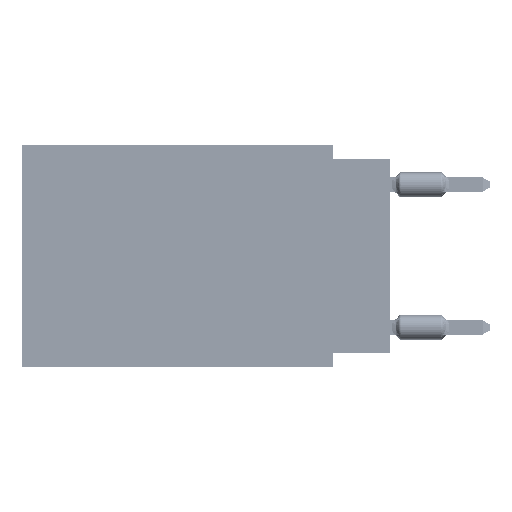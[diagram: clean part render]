
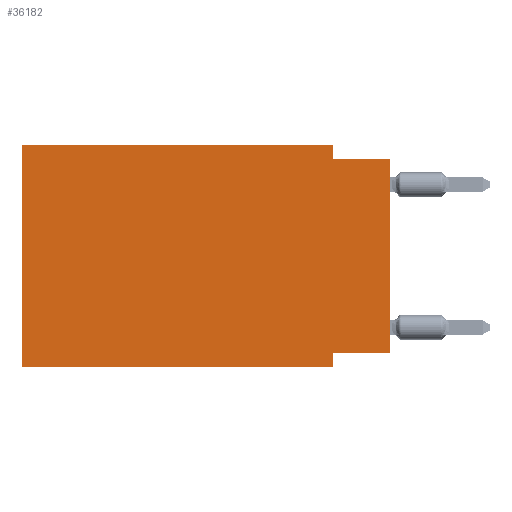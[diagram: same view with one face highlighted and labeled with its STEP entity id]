
A CAD part, left-side view. The second image highlights one B-rep face of the part: STEP entity #36182.
In plain terms, the highlighted planar face has unit normal (-1, 0, 0).
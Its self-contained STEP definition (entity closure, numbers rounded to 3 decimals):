
#5385 = CARTESIAN_POINT ( 'NONE',  ( 0., 2.54, 0. ) ) ;
#5853 = CARTESIAN_POINT ( 'NONE',  ( 0., 2.54, -9.906 ) ) ;
#7434 = EDGE_CURVE ( 'NONE', #43690, #29372, #51455, .T. ) ;
#8246 = DIRECTION ( 'NONE',  ( 0., 0., 1. ) ) ;
#9628 = DIRECTION ( 'NONE',  ( 0., 0., -1. ) ) ;
#9829 = EDGE_CURVE ( 'NONE', #29372, #57507, #38888, .T. ) ;
#11429 = EDGE_CURVE ( 'NONE', #43690, #33836, #52898, .T. ) ;
#11739 = CARTESIAN_POINT ( 'NONE',  ( 0., 16.383, 0. ) ) ;
#12144 = VERTEX_POINT ( 'NONE', #11739 ) ;
#13014 = VECTOR ( 'NONE', #66221, 1000. ) ;
#13335 = CARTESIAN_POINT ( 'NONE',  ( 0., 0., 0. ) ) ;
#14110 = DIRECTION ( 'NONE',  ( 0., -1., 0. ) ) ;
#15121 = VECTOR ( 'NONE', #14110, 1000. ) ;
#18585 = CARTESIAN_POINT ( 'NONE',  ( 0., 0., -9.271 ) ) ;
#19165 = VECTOR ( 'NONE', #28379, 1000. ) ;
#19522 = EDGE_CURVE ( 'NONE', #37060, #12144, #24349, .T. ) ;
#20546 = PLANE ( 'NONE',  #21403 ) ;
#20905 = ORIENTED_EDGE ( 'NONE', *, *, #7434, .F. ) ;
#21243 = VECTOR ( 'NONE', #57749, 1000. ) ;
#21403 = AXIS2_PLACEMENT_3D ( 'NONE', #70677, #31434, #9628 ) ;
#22285 = ORIENTED_EDGE ( 'NONE', *, *, #19522, .F. ) ;
#23385 = CARTESIAN_POINT ( 'NONE',  ( 0., 2.54, -0.635 ) ) ;
#24349 = LINE ( 'NONE', #35574, #21243 ) ;
#24928 = CARTESIAN_POINT ( 'NONE',  ( 0., 0., -0.635 ) ) ;
#26258 = VECTOR ( 'NONE', #8246, 1000. ) ;
#28379 = DIRECTION ( 'NONE',  ( 0., 0., -1. ) ) ;
#29372 = VERTEX_POINT ( 'NONE', #41130 ) ;
#31434 = DIRECTION ( 'NONE',  ( 1., 0., 0. ) ) ;
#33836 = VERTEX_POINT ( 'NONE', #62735 ) ;
#35095 = LINE ( 'NONE', #24928, #41537 ) ;
#35574 = CARTESIAN_POINT ( 'NONE',  ( 0., 16.383, 0. ) ) ;
#36182 = ADVANCED_FACE ( 'NONE', ( #53917 ), #20546, .F. ) ;
#37060 = VERTEX_POINT ( 'NONE', #42763 ) ;
#37344 = EDGE_CURVE ( 'NONE', #52095, #33836, #35095, .T. ) ;
#37492 = CARTESIAN_POINT ( 'NONE',  ( 0., 16.383, -9.906 ) ) ;
#37739 = ORIENTED_EDGE ( 'NONE', *, *, #9829, .F. ) ;
#38888 = LINE ( 'NONE', #5853, #19165 ) ;
#38912 = ORIENTED_EDGE ( 'NONE', *, *, #11429, .T. ) ;
#39270 = VERTEX_POINT ( 'NONE', #5385 ) ;
#41130 = CARTESIAN_POINT ( 'NONE',  ( 0., 2.54, -9.271 ) ) ;
#41537 = VECTOR ( 'NONE', #57251, 1000. ) ;
#41692 = LINE ( 'NONE', #63887, #15121 ) ;
#42763 = CARTESIAN_POINT ( 'NONE',  ( 0., 16.383, -9.906 ) ) ;
#43278 = DIRECTION ( 'NONE',  ( 0., -1., 0. ) ) ;
#43416 = EDGE_CURVE ( 'NONE', #37060, #57507, #59308, .T. ) ;
#43690 = VERTEX_POINT ( 'NONE', #18585 ) ;
#44213 = VECTOR ( 'NONE', #43278, 1000. ) ;
#46119 = ORIENTED_EDGE ( 'NONE', *, *, #54803, .F. ) ;
#47237 = CARTESIAN_POINT ( 'NONE',  ( 0., 2.54, -9.906 ) ) ;
#47550 = ORIENTED_EDGE ( 'NONE', *, *, #57164, .F. ) ;
#51119 = CARTESIAN_POINT ( 'NONE',  ( 0., 0., -9.271 ) ) ;
#51455 = LINE ( 'NONE', #51119, #61287 ) ;
#51520 = ORIENTED_EDGE ( 'NONE', *, *, #37344, .F. ) ;
#52095 = VERTEX_POINT ( 'NONE', #23385 ) ;
#52898 = LINE ( 'NONE', #13335, #26258 ) ;
#53917 = FACE_OUTER_BOUND ( 'NONE', #66120, .T. ) ;
#54803 = EDGE_CURVE ( 'NONE', #12144, #39270, #41692, .T. ) ;
#57164 = EDGE_CURVE ( 'NONE', #39270, #52095, #61468, .T. ) ;
#57251 = DIRECTION ( 'NONE',  ( 0., -1., 0. ) ) ;
#57507 = VERTEX_POINT ( 'NONE', #47237 ) ;
#57749 = DIRECTION ( 'NONE',  ( 0., 0., 1. ) ) ;
#59308 = LINE ( 'NONE', #37492, #44213 ) ;
#61285 = ORIENTED_EDGE ( 'NONE', *, *, #43416, .T. ) ;
#61287 = VECTOR ( 'NONE', #68920, 1000. ) ;
#61468 = LINE ( 'NONE', #66560, #13014 ) ;
#62735 = CARTESIAN_POINT ( 'NONE',  ( 0., 0., -0.635 ) ) ;
#63887 = CARTESIAN_POINT ( 'NONE',  ( 0., 16.383, 0. ) ) ;
#66120 = EDGE_LOOP ( 'NONE', ( #38912, #51520, #47550, #46119, #22285, #61285, #37739, #20905 ) ) ;
#66221 = DIRECTION ( 'NONE',  ( 0., 0., -1. ) ) ;
#66560 = CARTESIAN_POINT ( 'NONE',  ( 0., 2.54, 0. ) ) ;
#68920 = DIRECTION ( 'NONE',  ( 0., 1., 0. ) ) ;
#70677 = CARTESIAN_POINT ( 'NONE',  ( 0., 16.383, 0. ) ) ;
